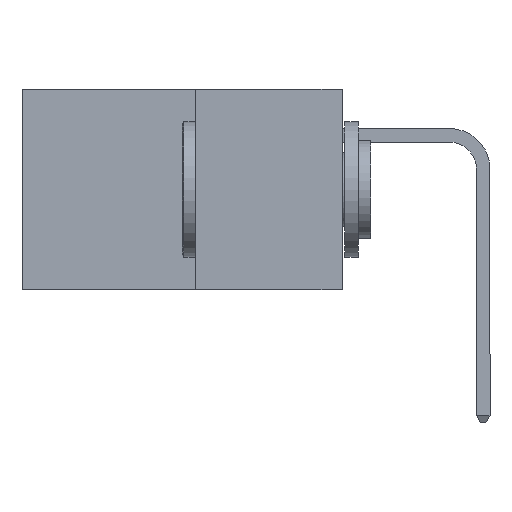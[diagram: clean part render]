
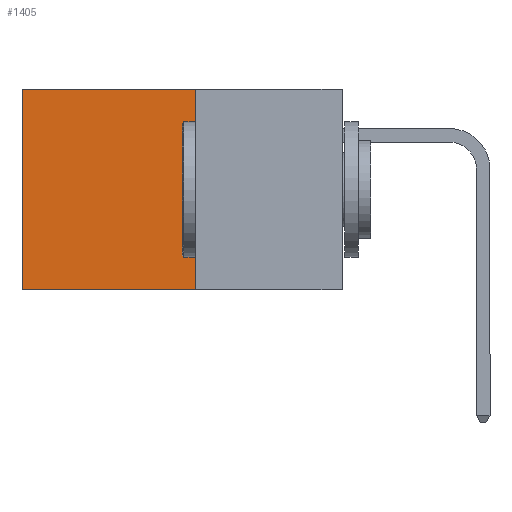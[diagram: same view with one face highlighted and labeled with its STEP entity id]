
A CAD part, left-side view. The second image highlights one B-rep face of the part: STEP entity #1405.
In plain terms, the highlighted planar face has unit normal (-1, 0, 0).
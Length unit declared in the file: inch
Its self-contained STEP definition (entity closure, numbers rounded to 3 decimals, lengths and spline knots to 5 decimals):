
#553 = VERTEX_POINT ( 'NONE', #16627 ) ;
#945 = VECTOR ( 'NONE', #2246, 39.37008 ) ;
#1200 = EDGE_CURVE ( 'NONE', #2629, #9369, #13763, .T. ) ;
#1405 = ADVANCED_FACE ( 'NONE', ( #3559 ), #9111, .F. ) ;
#2129 = CARTESIAN_POINT ( 'NONE',  ( 0.277, 0.27, 0. ) ) ;
#2246 = DIRECTION ( 'NONE',  ( 0., 1., 0. ) ) ;
#2325 = EDGE_CURVE ( 'NONE', #5749, #2629, #12666, .T. ) ;
#2629 = VERTEX_POINT ( 'NONE', #5279 ) ;
#3559 = FACE_OUTER_BOUND ( 'NONE', #16242, .T. ) ;
#4737 = DIRECTION ( 'NONE',  ( 0., 0., -1. ) ) ;
#4760 = CARTESIAN_POINT ( 'NONE',  ( 0.277, 0.27, -0.37 ) ) ;
#5087 = LINE ( 'NONE', #13106, #945 ) ;
#5221 = DIRECTION ( 'NONE',  ( 0., 0., -1. ) ) ;
#5279 = CARTESIAN_POINT ( 'NONE',  ( 0.277, 0.59, 0. ) ) ;
#5504 = VECTOR ( 'NONE', #13042, 39.37008 ) ;
#5749 = VERTEX_POINT ( 'NONE', #2129 ) ;
#6912 = ORIENTED_EDGE ( 'NONE', *, *, #7967, .F. ) ;
#7011 = CARTESIAN_POINT ( 'NONE',  ( 0.277, 0.27, -0.37 ) ) ;
#7967 = EDGE_CURVE ( 'NONE', #5749, #553, #13129, .T. ) ;
#8140 = AXIS2_PLACEMENT_3D ( 'NONE', #7011, #15174, #5221 ) ;
#9111 = PLANE ( 'NONE',  #8140 ) ;
#9369 = VERTEX_POINT ( 'NONE', #9867 ) ;
#9867 = CARTESIAN_POINT ( 'NONE',  ( 0.277, 0.59, -0.37 ) ) ;
#10258 = VECTOR ( 'NONE', #13286, 39.37008 ) ;
#10389 = CARTESIAN_POINT ( 'NONE',  ( 0.277, 0.27, 0. ) ) ;
#10841 = ORIENTED_EDGE ( 'NONE', *, *, #2325, .T. ) ;
#12666 = LINE ( 'NONE', #10389, #5504 ) ;
#13042 = DIRECTION ( 'NONE',  ( 0., 1., 0. ) ) ;
#13068 = EDGE_CURVE ( 'NONE', #553, #9369, #5087, .T. ) ;
#13106 = CARTESIAN_POINT ( 'NONE',  ( 0.277, 0.27, -0.37 ) ) ;
#13129 = LINE ( 'NONE', #4760, #17132 ) ;
#13286 = DIRECTION ( 'NONE',  ( 0., 0., -1. ) ) ;
#13763 = LINE ( 'NONE', #14763, #10258 ) ;
#14763 = CARTESIAN_POINT ( 'NONE',  ( 0.277, 0.59, -0.37 ) ) ;
#15174 = DIRECTION ( 'NONE',  ( 1., 0., 0. ) ) ;
#16242 = EDGE_LOOP ( 'NONE', ( #16690, #17114, #6912, #10841 ) ) ;
#16627 = CARTESIAN_POINT ( 'NONE',  ( 0.277, 0.27, -0.37 ) ) ;
#16690 = ORIENTED_EDGE ( 'NONE', *, *, #1200, .T. ) ;
#17114 = ORIENTED_EDGE ( 'NONE', *, *, #13068, .F. ) ;
#17132 = VECTOR ( 'NONE', #4737, 39.37008 ) ;
